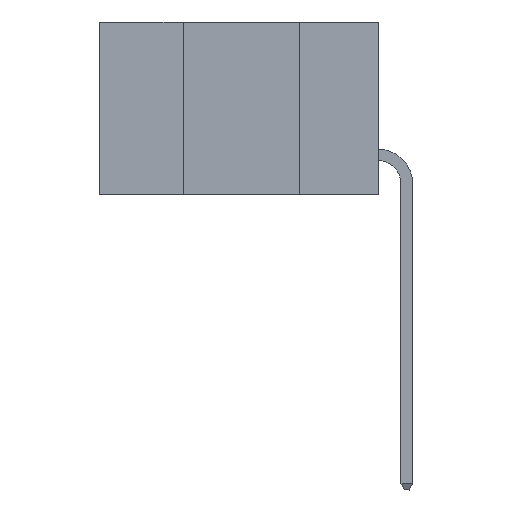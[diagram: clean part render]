
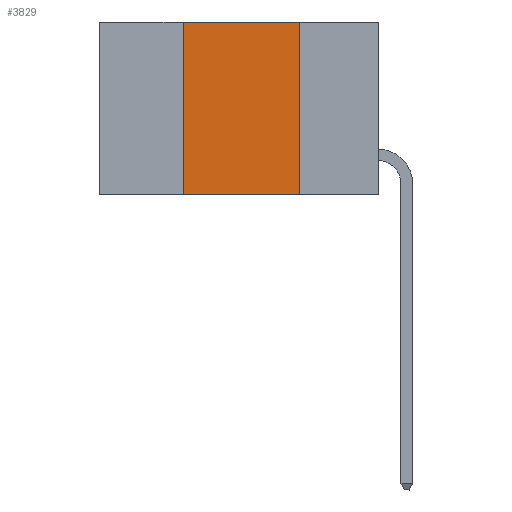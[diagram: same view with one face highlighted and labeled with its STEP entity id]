
A CAD part, left-side view. The second image highlights one B-rep face of the part: STEP entity #3829.
In plain terms, the highlighted planar face has unit normal (-1, 0, 0).
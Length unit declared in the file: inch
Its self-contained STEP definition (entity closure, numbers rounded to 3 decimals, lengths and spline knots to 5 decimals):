
#157 = CARTESIAN_POINT ( 'NONE',  ( 0., 0.42, -0.37 ) ) ;
#516 = PLANE ( 'NONE',  #1611 ) ;
#721 = ORIENTED_EDGE ( 'NONE', *, *, #11029, .F. ) ;
#756 = EDGE_CURVE ( 'NONE', #7847, #6261, #8883, .T. ) ;
#1478 = DIRECTION ( 'NONE',  ( 0., 0., -1. ) ) ;
#1534 = FACE_OUTER_BOUND ( 'NONE', #8845, .T. ) ;
#1577 = ORIENTED_EDGE ( 'NONE', *, *, #4682, .F. ) ;
#1611 = AXIS2_PLACEMENT_3D ( 'NONE', #5651, #4807, #1478 ) ;
#2036 = DIRECTION ( 'NONE',  ( 0., 0., -1. ) ) ;
#2099 = CARTESIAN_POINT ( 'NONE',  ( 0., 0.17, 0. ) ) ;
#2387 = EDGE_CURVE ( 'NONE', #3833, #6261, #4729, .T. ) ;
#2977 = DIRECTION ( 'NONE',  ( 0., -1., 0. ) ) ;
#3626 = DIRECTION ( 'NONE',  ( 0., 0., 1. ) ) ;
#3680 = ORIENTED_EDGE ( 'NONE', *, *, #2387, .T. ) ;
#3829 = ADVANCED_FACE ( 'NONE', ( #1534 ), #516, .F. ) ;
#3833 = VERTEX_POINT ( 'NONE', #8265 ) ;
#4422 = LINE ( 'NONE', #157, #9309 ) ;
#4632 = CARTESIAN_POINT ( 'NONE',  ( 0., 0.17, -0.37 ) ) ;
#4682 = EDGE_CURVE ( 'NONE', #8280, #7847, #10817, .T. ) ;
#4729 = LINE ( 'NONE', #5522, #10988 ) ;
#4807 = DIRECTION ( 'NONE',  ( 1., 0., 0. ) ) ;
#5522 = CARTESIAN_POINT ( 'NONE',  ( 0., 0.6, -0.37 ) ) ;
#5651 = CARTESIAN_POINT ( 'NONE',  ( 0., 0.6, 0. ) ) ;
#5837 = CARTESIAN_POINT ( 'NONE',  ( 0., 0.6, 0. ) ) ;
#6261 = VERTEX_POINT ( 'NONE', #6622 ) ;
#6622 = CARTESIAN_POINT ( 'NONE',  ( 0., 0.17, -0.37 ) ) ;
#6630 = VECTOR ( 'NONE', #8399, 39.37008 ) ;
#7847 = VERTEX_POINT ( 'NONE', #2099 ) ;
#8265 = CARTESIAN_POINT ( 'NONE',  ( 0., 0.42, -0.37 ) ) ;
#8280 = VERTEX_POINT ( 'NONE', #9698 ) ;
#8399 = DIRECTION ( 'NONE',  ( 0., -1., 0. ) ) ;
#8845 = EDGE_LOOP ( 'NONE', ( #10840, #1577, #721, #3680 ) ) ;
#8883 = LINE ( 'NONE', #4632, #9288 ) ;
#9288 = VECTOR ( 'NONE', #2036, 39.37008 ) ;
#9309 = VECTOR ( 'NONE', #3626, 39.37008 ) ;
#9698 = CARTESIAN_POINT ( 'NONE',  ( 0., 0.42, 0. ) ) ;
#10817 = LINE ( 'NONE', #5837, #6630 ) ;
#10840 = ORIENTED_EDGE ( 'NONE', *, *, #756, .F. ) ;
#10988 = VECTOR ( 'NONE', #2977, 39.37008 ) ;
#11029 = EDGE_CURVE ( 'NONE', #3833, #8280, #4422, .T. ) ;
